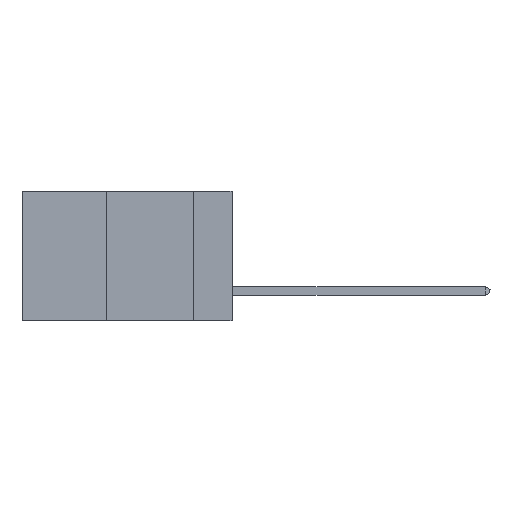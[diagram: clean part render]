
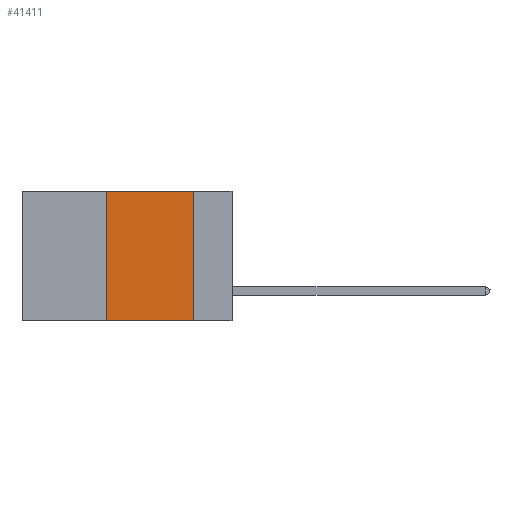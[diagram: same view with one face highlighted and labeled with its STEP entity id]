
A CAD part, left-side view. The second image highlights one B-rep face of the part: STEP entity #41411.
In plain terms, the highlighted planar face has unit normal (-1, 0, 0).
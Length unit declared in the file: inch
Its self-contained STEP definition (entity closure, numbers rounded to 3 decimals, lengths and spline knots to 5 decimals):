
#28 = CARTESIAN_POINT ( 'NONE',  ( 0., 0.11, -0.37 ) ) ;
#1190 = VECTOR ( 'NONE', #4076, 39.37008 ) ;
#2758 = ORIENTED_EDGE ( 'NONE', *, *, #26703, .T. ) ;
#3803 = ORIENTED_EDGE ( 'NONE', *, *, #10356, .F. ) ;
#4076 = DIRECTION ( 'NONE',  ( 0., -1., 0. ) ) ;
#4150 = FACE_OUTER_BOUND ( 'NONE', #44125, .T. ) ;
#4380 = DIRECTION ( 'NONE',  ( 0., 0., -1. ) ) ;
#4598 = DIRECTION ( 'NONE',  ( 1., 0., 0. ) ) ;
#5076 = VERTEX_POINT ( 'NONE', #25269 ) ;
#6958 = EDGE_CURVE ( 'NONE', #39183, #21205, #40051, .T. ) ;
#10356 = EDGE_CURVE ( 'NONE', #5076, #30646, #30985, .T. ) ;
#11812 = PLANE ( 'NONE',  #21400 ) ;
#17907 = CARTESIAN_POINT ( 'NONE',  ( 0., 0.6, 0. ) ) ;
#19961 = CARTESIAN_POINT ( 'NONE',  ( 0., 0.6, -0.37 ) ) ;
#20016 = CARTESIAN_POINT ( 'NONE',  ( 0., 0.36, 0. ) ) ;
#21205 = VERTEX_POINT ( 'NONE', #29543 ) ;
#21210 = LINE ( 'NONE', #41928, #1190 ) ;
#21400 = AXIS2_PLACEMENT_3D ( 'NONE', #17907, #4598, #4380 ) ;
#23126 = LINE ( 'NONE', #19961, #44007 ) ;
#24889 = CARTESIAN_POINT ( 'NONE',  ( 0., 0.11, 0. ) ) ;
#25269 = CARTESIAN_POINT ( 'NONE',  ( 0., 0.11, 0. ) ) ;
#25655 = VECTOR ( 'NONE', #41112, 39.37008 ) ;
#26703 = EDGE_CURVE ( 'NONE', #39183, #30646, #23126, .T. ) ;
#29290 = VECTOR ( 'NONE', #37562, 39.37008 ) ;
#29543 = CARTESIAN_POINT ( 'NONE',  ( 0., 0.36, 0. ) ) ;
#30646 = VERTEX_POINT ( 'NONE', #28 ) ;
#30985 = LINE ( 'NONE', #24889, #25655 ) ;
#31221 = CARTESIAN_POINT ( 'NONE',  ( 0., 0.36, -0.37 ) ) ;
#33131 = ORIENTED_EDGE ( 'NONE', *, *, #6958, .F. ) ;
#33479 = DIRECTION ( 'NONE',  ( 0., -1., 0. ) ) ;
#34443 = ORIENTED_EDGE ( 'NONE', *, *, #39952, .F. ) ;
#37562 = DIRECTION ( 'NONE',  ( 0., 0., 1. ) ) ;
#39183 = VERTEX_POINT ( 'NONE', #31221 ) ;
#39952 = EDGE_CURVE ( 'NONE', #21205, #5076, #21210, .T. ) ;
#40051 = LINE ( 'NONE', #20016, #29290 ) ;
#41112 = DIRECTION ( 'NONE',  ( 0., 0., -1. ) ) ;
#41411 = ADVANCED_FACE ( 'NONE', ( #4150 ), #11812, .F. ) ;
#41928 = CARTESIAN_POINT ( 'NONE',  ( 0., 0.6, 0. ) ) ;
#44007 = VECTOR ( 'NONE', #33479, 39.37008 ) ;
#44125 = EDGE_LOOP ( 'NONE', ( #3803, #34443, #33131, #2758 ) ) ;
